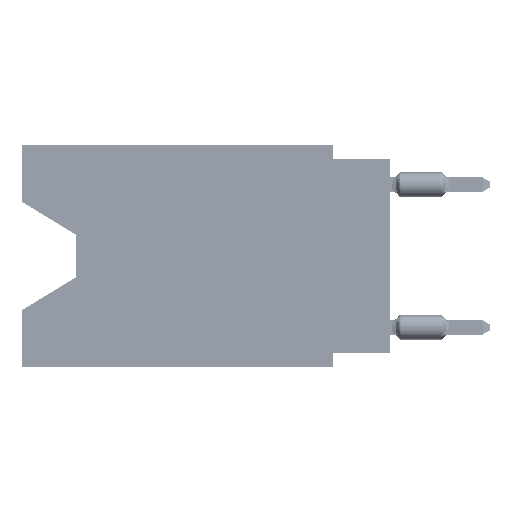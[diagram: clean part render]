
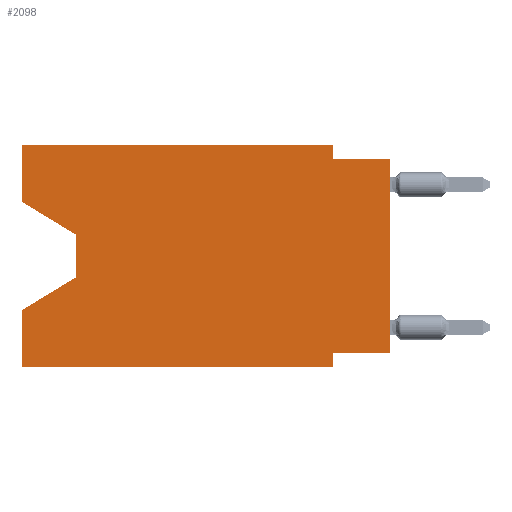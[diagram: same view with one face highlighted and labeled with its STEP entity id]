
A CAD part, left-side view. The second image highlights one B-rep face of the part: STEP entity #2098.
In plain terms, the highlighted planar face has unit normal (-1, 0, 0).
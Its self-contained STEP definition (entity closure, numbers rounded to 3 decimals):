
#661 = LINE ( 'NONE', #40577, #24046 ) ;
#1393 = EDGE_CURVE ( 'NONE', #50931, #65856, #60192, .T. ) ;
#1613 = CARTESIAN_POINT ( 'NONE',  ( 0., 0., -0.635 ) ) ;
#2098 = ADVANCED_FACE ( 'NONE', ( #33041 ), #18731, .F. ) ;
#2117 = CARTESIAN_POINT ( 'NONE',  ( 0., 16.383, -2.546 ) ) ;
#2122 = CARTESIAN_POINT ( 'NONE',  ( 0., 16.383, -9.906 ) ) ;
#3059 = LINE ( 'NONE', #3918, #21767 ) ;
#3918 = CARTESIAN_POINT ( 'NONE',  ( 0., 13.97, -4.013 ) ) ;
#4925 = ORIENTED_EDGE ( 'NONE', *, *, #45424, .T. ) ;
#4979 = VECTOR ( 'NONE', #18258, 1000. ) ;
#5228 = DIRECTION ( 'NONE',  ( 0., 0., -1. ) ) ;
#5855 = CARTESIAN_POINT ( 'NONE',  ( 0., 2.54, -0.635 ) ) ;
#7850 = DIRECTION ( 'NONE',  ( 0., 0.855, -0.519 ) ) ;
#9592 = DIRECTION ( 'NONE',  ( 0., 0., -1. ) ) ;
#11240 = EDGE_LOOP ( 'NONE', ( #4925, #42777, #84481, #43742, #29132, #49485, #61232, #85305, #25526, #13081, #35688, #15446 ) ) ;
#12748 = VERTEX_POINT ( 'NONE', #42045 ) ;
#13081 = ORIENTED_EDGE ( 'NONE', *, *, #14518, .F. ) ;
#14518 = EDGE_CURVE ( 'NONE', #12748, #37432, #64737, .T. ) ;
#15156 = LINE ( 'NONE', #2122, #84108 ) ;
#15446 = ORIENTED_EDGE ( 'NONE', *, *, #1393, .F. ) ;
#18258 = DIRECTION ( 'NONE',  ( 0., -1., 0. ) ) ;
#18731 = PLANE ( 'NONE',  #84512 ) ;
#19134 = CARTESIAN_POINT ( 'NONE',  ( 0., 2.54, -9.906 ) ) ;
#19560 = CARTESIAN_POINT ( 'NONE',  ( 0., 16.383, 0. ) ) ;
#19978 = DIRECTION ( 'NONE',  ( 0., -1., 0. ) ) ;
#20271 = DIRECTION ( 'NONE',  ( 0., 0., 1. ) ) ;
#21767 = VECTOR ( 'NONE', #9592, 1000. ) ;
#23999 = EDGE_CURVE ( 'NONE', #34121, #56340, #66003, .T. ) ;
#24046 = VECTOR ( 'NONE', #27157, 1000. ) ;
#24483 = LINE ( 'NONE', #1613, #61510 ) ;
#24698 = VECTOR ( 'NONE', #59911, 1000. ) ;
#24803 = CARTESIAN_POINT ( 'NONE',  ( 0., 2.54, 0. ) ) ;
#25526 = ORIENTED_EDGE ( 'NONE', *, *, #82261, .F. ) ;
#26061 = CARTESIAN_POINT ( 'NONE',  ( 0., 16.383, 0. ) ) ;
#26073 = LINE ( 'NONE', #19134, #72004 ) ;
#26992 = LINE ( 'NONE', #67357, #56873 ) ;
#27157 = DIRECTION ( 'NONE',  ( 0., 1., 0. ) ) ;
#29132 = ORIENTED_EDGE ( 'NONE', *, *, #34764, .T. ) ;
#30207 = CARTESIAN_POINT ( 'NONE',  ( 0., 16.383, 0. ) ) ;
#33041 = FACE_OUTER_BOUND ( 'NONE', #11240, .T. ) ;
#33364 = DIRECTION ( 'NONE',  ( 0., 0., 1. ) ) ;
#34121 = VERTEX_POINT ( 'NONE', #50932 ) ;
#34595 = EDGE_CURVE ( 'NONE', #65856, #12748, #51675, .T. ) ;
#34764 = EDGE_CURVE ( 'NONE', #34121, #37862, #15156, .T. ) ;
#35688 = ORIENTED_EDGE ( 'NONE', *, *, #34595, .F. ) ;
#35888 = DIRECTION ( 'NONE',  ( 0., -1., 0. ) ) ;
#37432 = VERTEX_POINT ( 'NONE', #5855 ) ;
#37862 = VERTEX_POINT ( 'NONE', #71353 ) ;
#38217 = EDGE_CURVE ( 'NONE', #52812, #37862, #26073, .T. ) ;
#38639 = DIRECTION ( 'NONE',  ( 0., 0., -1. ) ) ;
#39960 = DIRECTION ( 'NONE',  ( 1., 0., 0. ) ) ;
#40577 = CARTESIAN_POINT ( 'NONE',  ( 0., 0., -9.271 ) ) ;
#41821 = VERTEX_POINT ( 'NONE', #51621 ) ;
#42045 = CARTESIAN_POINT ( 'NONE',  ( 0., 2.54, 0. ) ) ;
#42777 = ORIENTED_EDGE ( 'NONE', *, *, #74312, .T. ) ;
#43158 = CARTESIAN_POINT ( 'NONE',  ( 0., 13.97, -4.013 ) ) ;
#43742 = ORIENTED_EDGE ( 'NONE', *, *, #23999, .F. ) ;
#43840 = EDGE_CURVE ( 'NONE', #41821, #56340, #26992, .T. ) ;
#45424 = EDGE_CURVE ( 'NONE', #50931, #77718, #81525, .T. ) ;
#45518 = CARTESIAN_POINT ( 'NONE',  ( 0., 16.383, -7.36 ) ) ;
#45557 = VECTOR ( 'NONE', #20271, 1000. ) ;
#45781 = EDGE_CURVE ( 'NONE', #72495, #52812, #661, .T. ) ;
#46271 = VERTEX_POINT ( 'NONE', #82160 ) ;
#49349 = DIRECTION ( 'NONE',  ( 0., -0.855, -0.519 ) ) ;
#49485 = ORIENTED_EDGE ( 'NONE', *, *, #38217, .F. ) ;
#50806 = CARTESIAN_POINT ( 'NONE',  ( 0., 2.54, -9.271 ) ) ;
#50931 = VERTEX_POINT ( 'NONE', #2117 ) ;
#50932 = CARTESIAN_POINT ( 'NONE',  ( 0., 16.383, -9.906 ) ) ;
#51621 = CARTESIAN_POINT ( 'NONE',  ( 0., 13.97, -5.893 ) ) ;
#51675 = LINE ( 'NONE', #26061, #4979 ) ;
#52812 = VERTEX_POINT ( 'NONE', #50806 ) ;
#56340 = VERTEX_POINT ( 'NONE', #45518 ) ;
#56873 = VECTOR ( 'NONE', #7850, 1000. ) ;
#58621 = VECTOR ( 'NONE', #49349, 1000. ) ;
#59911 = DIRECTION ( 'NONE',  ( 0., 0., 1. ) ) ;
#60192 = LINE ( 'NONE', #73252, #45557 ) ;
#61232 = ORIENTED_EDGE ( 'NONE', *, *, #45781, .F. ) ;
#61510 = VECTOR ( 'NONE', #35888, 1000. ) ;
#64698 = VECTOR ( 'NONE', #33364, 1000. ) ;
#64737 = LINE ( 'NONE', #24803, #72185 ) ;
#65856 = VERTEX_POINT ( 'NONE', #30207 ) ;
#65923 = LINE ( 'NONE', #74150, #64698 ) ;
#66003 = LINE ( 'NONE', #19560, #24698 ) ;
#67357 = CARTESIAN_POINT ( 'NONE',  ( 0., 13.97, -5.893 ) ) ;
#68476 = CARTESIAN_POINT ( 'NONE',  ( 0., 16.383, -2.546 ) ) ;
#69209 = CARTESIAN_POINT ( 'NONE',  ( 0., 0., -9.271 ) ) ;
#71353 = CARTESIAN_POINT ( 'NONE',  ( 0., 2.54, -9.906 ) ) ;
#71709 = DIRECTION ( 'NONE',  ( 0., 0., -1. ) ) ;
#72004 = VECTOR ( 'NONE', #38639, 1000. ) ;
#72185 = VECTOR ( 'NONE', #5228, 1000. ) ;
#72495 = VERTEX_POINT ( 'NONE', #69209 ) ;
#73252 = CARTESIAN_POINT ( 'NONE',  ( 0., 16.383, 0. ) ) ;
#74150 = CARTESIAN_POINT ( 'NONE',  ( 0., 0., 0. ) ) ;
#74312 = EDGE_CURVE ( 'NONE', #77718, #41821, #3059, .T. ) ;
#77718 = VERTEX_POINT ( 'NONE', #43158 ) ;
#79073 = CARTESIAN_POINT ( 'NONE',  ( 0., 16.383, 0. ) ) ;
#81525 = LINE ( 'NONE', #68476, #58621 ) ;
#82160 = CARTESIAN_POINT ( 'NONE',  ( 0., 0., -0.635 ) ) ;
#82261 = EDGE_CURVE ( 'NONE', #37432, #46271, #24483, .T. ) ;
#83289 = EDGE_CURVE ( 'NONE', #72495, #46271, #65923, .T. ) ;
#84108 = VECTOR ( 'NONE', #19978, 1000. ) ;
#84481 = ORIENTED_EDGE ( 'NONE', *, *, #43840, .T. ) ;
#84512 = AXIS2_PLACEMENT_3D ( 'NONE', #79073, #39960, #71709 ) ;
#85305 = ORIENTED_EDGE ( 'NONE', *, *, #83289, .T. ) ;
